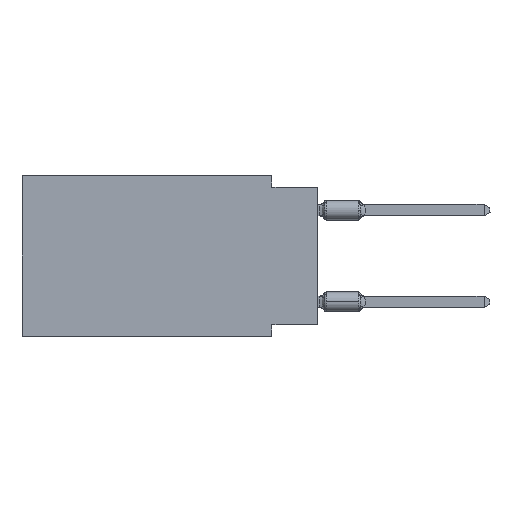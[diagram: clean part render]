
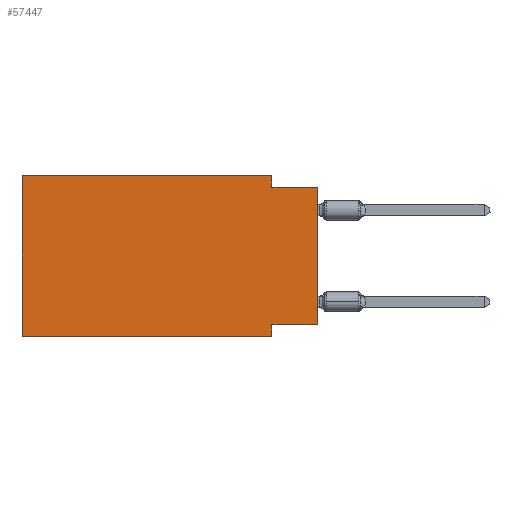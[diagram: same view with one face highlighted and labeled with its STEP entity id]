
A CAD part, left-side view. The second image highlights one B-rep face of the part: STEP entity #57447.
In plain terms, the highlighted planar face has unit normal (-1, 0, 0).
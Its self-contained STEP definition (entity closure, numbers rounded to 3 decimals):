
#894 = ORIENTED_EDGE ( 'NONE', *, *, #31057, .T. ) ;
#2219 = VERTEX_POINT ( 'NONE', #12540 ) ;
#3028 = VERTEX_POINT ( 'NONE', #3228 ) ;
#3228 = CARTESIAN_POINT ( 'NONE',  ( 0., 2.54, -8.255 ) ) ;
#3867 = LINE ( 'NONE', #59012, #45156 ) ;
#3930 = VERTEX_POINT ( 'NONE', #19636 ) ;
#4074 = CARTESIAN_POINT ( 'NONE',  ( 0., 16.383, -8.89 ) ) ;
#5866 = CARTESIAN_POINT ( 'NONE',  ( 0., 0., -0.635 ) ) ;
#7905 = LINE ( 'NONE', #46729, #46305 ) ;
#8336 = DIRECTION ( 'NONE',  ( 1., 0., 0. ) ) ;
#10902 = VECTOR ( 'NONE', #50428, 1000. ) ;
#11411 = VERTEX_POINT ( 'NONE', #57087 ) ;
#12540 = CARTESIAN_POINT ( 'NONE',  ( 0., 16.383, 0. ) ) ;
#13452 = CARTESIAN_POINT ( 'NONE',  ( 0., 2.54, -0.635 ) ) ;
#14133 = EDGE_CURVE ( 'NONE', #3028, #3930, #34679, .T. ) ;
#14515 = ORIENTED_EDGE ( 'NONE', *, *, #57526, .F. ) ;
#14535 = DIRECTION ( 'NONE',  ( 0., -1., 0. ) ) ;
#14684 = ORIENTED_EDGE ( 'NONE', *, *, #14133, .F. ) ;
#14772 = DIRECTION ( 'NONE',  ( 0., 0., -1. ) ) ;
#17398 = CARTESIAN_POINT ( 'NONE',  ( 0., 0., -8.255 ) ) ;
#19636 = CARTESIAN_POINT ( 'NONE',  ( 0., 2.54, -8.89 ) ) ;
#22563 = EDGE_CURVE ( 'NONE', #57435, #2219, #30230, .T. ) ;
#23104 = AXIS2_PLACEMENT_3D ( 'NONE', #62838, #8336, #58894 ) ;
#24414 = VERTEX_POINT ( 'NONE', #17398 ) ;
#26436 = CARTESIAN_POINT ( 'NONE',  ( 0., 0., -8.255 ) ) ;
#26803 = DIRECTION ( 'NONE',  ( 0., 0., -1. ) ) ;
#27821 = DIRECTION ( 'NONE',  ( 0., -1., 0. ) ) ;
#27934 = FACE_OUTER_BOUND ( 'NONE', #59376, .T. ) ;
#29362 = EDGE_CURVE ( 'NONE', #31151, #48930, #3867, .T. ) ;
#30230 = LINE ( 'NONE', #55316, #10902 ) ;
#30634 = DIRECTION ( 'NONE',  ( 0., 0., 1. ) ) ;
#31057 = EDGE_CURVE ( 'NONE', #57435, #3930, #7905, .T. ) ;
#31151 = VERTEX_POINT ( 'NONE', #13452 ) ;
#31606 = LINE ( 'NONE', #50825, #36214 ) ;
#33590 = DIRECTION ( 'NONE',  ( 0., -1., 0. ) ) ;
#33665 = ORIENTED_EDGE ( 'NONE', *, *, #22563, .F. ) ;
#34679 = LINE ( 'NONE', #53893, #36184 ) ;
#35041 = EDGE_CURVE ( 'NONE', #24414, #3028, #35565, .T. ) ;
#35081 = CARTESIAN_POINT ( 'NONE',  ( 0., 16.383, 0. ) ) ;
#35565 = LINE ( 'NONE', #26436, #51857 ) ;
#36184 = VECTOR ( 'NONE', #14772, 1000. ) ;
#36214 = VECTOR ( 'NONE', #30634, 1000. ) ;
#37212 = LINE ( 'NONE', #41782, #55308 ) ;
#38946 = EDGE_CURVE ( 'NONE', #11411, #31151, #37212, .T. ) ;
#40766 = ORIENTED_EDGE ( 'NONE', *, *, #38946, .F. ) ;
#41100 = DIRECTION ( 'NONE',  ( 0., 1., 0. ) ) ;
#41766 = EDGE_CURVE ( 'NONE', #24414, #48930, #31606, .T. ) ;
#41782 = CARTESIAN_POINT ( 'NONE',  ( 0., 2.54, 0. ) ) ;
#42147 = ORIENTED_EDGE ( 'NONE', *, *, #35041, .F. ) ;
#45156 = VECTOR ( 'NONE', #33590, 1000. ) ;
#46305 = VECTOR ( 'NONE', #27821, 1000. ) ;
#46729 = CARTESIAN_POINT ( 'NONE',  ( 0., 16.383, -8.89 ) ) ;
#47804 = PLANE ( 'NONE',  #23104 ) ;
#48930 = VERTEX_POINT ( 'NONE', #5866 ) ;
#50428 = DIRECTION ( 'NONE',  ( 0., 0., 1. ) ) ;
#50825 = CARTESIAN_POINT ( 'NONE',  ( 0., 0., 0. ) ) ;
#51857 = VECTOR ( 'NONE', #41100, 1000. ) ;
#53893 = CARTESIAN_POINT ( 'NONE',  ( 0., 2.54, -8.89 ) ) ;
#55308 = VECTOR ( 'NONE', #26803, 1000. ) ;
#55316 = CARTESIAN_POINT ( 'NONE',  ( 0., 16.383, 0. ) ) ;
#57087 = CARTESIAN_POINT ( 'NONE',  ( 0., 2.54, 0. ) ) ;
#57435 = VERTEX_POINT ( 'NONE', #4074 ) ;
#57447 = ADVANCED_FACE ( 'NONE', ( #27934 ), #47804, .F. ) ;
#57471 = VECTOR ( 'NONE', #14535, 1000. ) ;
#57526 = EDGE_CURVE ( 'NONE', #2219, #11411, #59867, .T. ) ;
#58894 = DIRECTION ( 'NONE',  ( 0., 0., -1. ) ) ;
#59012 = CARTESIAN_POINT ( 'NONE',  ( 0., 0., -0.635 ) ) ;
#59376 = EDGE_LOOP ( 'NONE', ( #60494, #62573, #40766, #14515, #33665, #894, #14684, #42147 ) ) ;
#59867 = LINE ( 'NONE', #35081, #57471 ) ;
#60494 = ORIENTED_EDGE ( 'NONE', *, *, #41766, .T. ) ;
#62573 = ORIENTED_EDGE ( 'NONE', *, *, #29362, .F. ) ;
#62838 = CARTESIAN_POINT ( 'NONE',  ( 0., 16.383, 0. ) ) ;
